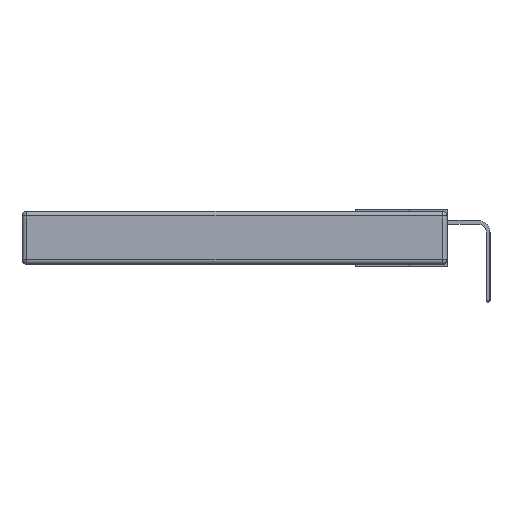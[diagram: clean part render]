
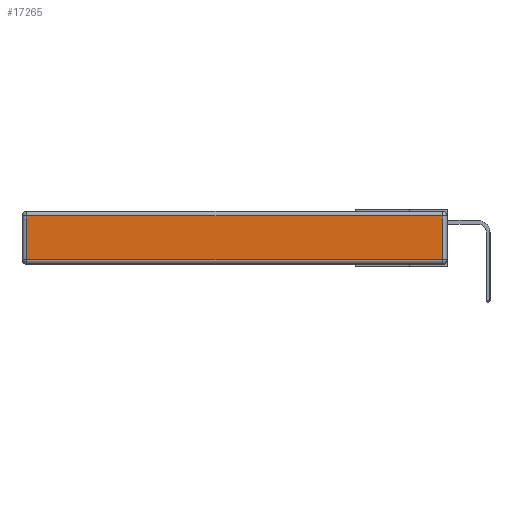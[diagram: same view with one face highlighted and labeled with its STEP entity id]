
A CAD part, left-side view. The second image highlights one B-rep face of the part: STEP entity #17265.
In plain terms, the highlighted planar face has unit normal (-1, 0, 0).
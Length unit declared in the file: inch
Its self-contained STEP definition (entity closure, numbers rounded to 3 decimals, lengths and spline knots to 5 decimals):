
#166 = PLANE ( 'NONE',  #1805 ) ;
#643 = EDGE_CURVE ( 'NONE', #14782, #1864, #10271, .T. ) ;
#788 = CARTESIAN_POINT ( 'NONE',  ( 0., 0.03, -0.313 ) ) ;
#1323 = DIRECTION ( 'NONE',  ( 0., -1., 0. ) ) ;
#1358 = ORIENTED_EDGE ( 'NONE', *, *, #12676, .T. ) ;
#1599 = VECTOR ( 'NONE', #16353, 39.37008 ) ;
#1805 = AXIS2_PLACEMENT_3D ( 'NONE', #11684, #6862, #13638 ) ;
#1864 = VERTEX_POINT ( 'NONE', #13539 ) ;
#2371 = DIRECTION ( 'NONE',  ( 0., 1., 0. ) ) ;
#3208 = CARTESIAN_POINT ( 'NONE',  ( 0., 0.03, -0.343 ) ) ;
#4835 = ORIENTED_EDGE ( 'NONE', *, *, #14768, .T. ) ;
#5676 = VECTOR ( 'NONE', #2371, 39.37008 ) ;
#6483 = CARTESIAN_POINT ( 'NONE',  ( 0., 0.03, -0.03 ) ) ;
#6862 = DIRECTION ( 'NONE',  ( -1., 0., 0. ) ) ;
#7624 = ORIENTED_EDGE ( 'NONE', *, *, #643, .T. ) ;
#8872 = LINE ( 'NONE', #20867, #15307 ) ;
#9365 = DIRECTION ( 'NONE',  ( 0., 0., -1. ) ) ;
#10271 = LINE ( 'NONE', #13847, #5676 ) ;
#11621 = LINE ( 'NONE', #3208, #1599 ) ;
#11684 = CARTESIAN_POINT ( 'NONE',  ( 0., 0., -0.343 ) ) ;
#12676 = EDGE_CURVE ( 'NONE', #16226, #14782, #11621, .T. ) ;
#13539 = CARTESIAN_POINT ( 'NONE',  ( 0., 2.72, -0.03 ) ) ;
#13638 = DIRECTION ( 'NONE',  ( 0., 0., 1. ) ) ;
#13847 = CARTESIAN_POINT ( 'NONE',  ( 0., 2.75, -0.03 ) ) ;
#14068 = VERTEX_POINT ( 'NONE', #17798 ) ;
#14768 = EDGE_CURVE ( 'NONE', #1864, #14068, #8872, .T. ) ;
#14782 = VERTEX_POINT ( 'NONE', #6483 ) ;
#15307 = VECTOR ( 'NONE', #9365, 39.37008 ) ;
#16226 = VERTEX_POINT ( 'NONE', #788 ) ;
#16353 = DIRECTION ( 'NONE',  ( 0., 0., 1. ) ) ;
#17079 = FACE_OUTER_BOUND ( 'NONE', #18706, .T. ) ;
#17265 = ADVANCED_FACE ( 'NONE', ( #17079 ), #166, .T. ) ;
#17629 = CARTESIAN_POINT ( 'NONE',  ( 0., 0., -0.313 ) ) ;
#17798 = CARTESIAN_POINT ( 'NONE',  ( 0., 2.72, -0.313 ) ) ;
#18706 = EDGE_LOOP ( 'NONE', ( #19262, #1358, #7624, #4835 ) ) ;
#18781 = EDGE_CURVE ( 'NONE', #14068, #16226, #19817, .T. ) ;
#19262 = ORIENTED_EDGE ( 'NONE', *, *, #18781, .T. ) ;
#19817 = LINE ( 'NONE', #17629, #20823 ) ;
#20823 = VECTOR ( 'NONE', #1323, 39.37008 ) ;
#20867 = CARTESIAN_POINT ( 'NONE',  ( 0., 2.72, -0.343 ) ) ;
